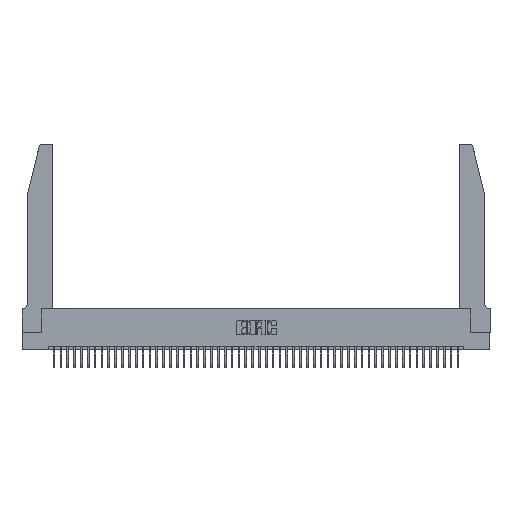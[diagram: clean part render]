
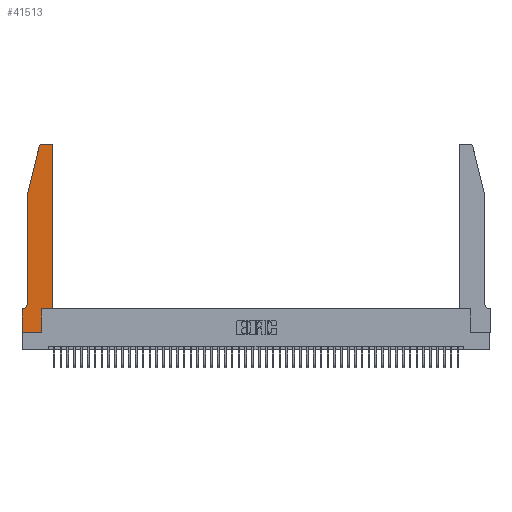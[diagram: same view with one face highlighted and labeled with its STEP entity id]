
A CAD part, top view. The second image highlights one B-rep face of the part: STEP entity #41513.
In plain terms, the highlighted planar face has unit normal (0, 0, 1).
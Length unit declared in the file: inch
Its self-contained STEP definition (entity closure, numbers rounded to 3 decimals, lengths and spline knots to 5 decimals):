
#330 = CIRCLE ( 'NONE', #25915, 0.07 ) ;
#775 = VECTOR ( 'NONE', #23107, 39.37008 ) ;
#2225 = VECTOR ( 'NONE', #41703, 39.37008 ) ;
#2553 = VERTEX_POINT ( 'NONE', #5997 ) ;
#3724 = CARTESIAN_POINT ( 'NONE',  ( 0., 0., 0.37 ) ) ;
#4008 = ORIENTED_EDGE ( 'NONE', *, *, #17469, .T. ) ;
#4079 = ORIENTED_EDGE ( 'NONE', *, *, #15821, .T. ) ;
#4320 = DIRECTION ( 'NONE',  ( 0., 0., 1. ) ) ;
#4356 = VERTEX_POINT ( 'NONE', #34598 ) ;
#4429 = PLANE ( 'NONE',  #10788 ) ;
#4528 = DIRECTION ( 'NONE',  ( -1., 0., 0. ) ) ;
#4863 = CARTESIAN_POINT ( 'NONE',  ( 0.0755, 2., 0.37 ) ) ;
#4899 = LINE ( 'NONE', #30300, #35871 ) ;
#5863 = DIRECTION ( 'NONE',  ( 0., 0., -1. ) ) ;
#5871 = EDGE_CURVE ( 'NONE', #2553, #21811, #7410, .T. ) ;
#5997 = CARTESIAN_POINT ( 'NONE',  ( 0.4205, 2.75, 0.37 ) ) ;
#6788 = VERTEX_POINT ( 'NONE', #37361 ) ;
#7410 = LINE ( 'NONE', #32541, #9270 ) ;
#7857 = EDGE_CURVE ( 'NONE', #38360, #44325, #42162, .T. ) ;
#8050 = LINE ( 'NONE', #15309, #49003 ) ;
#8825 = DIRECTION ( 'NONE',  ( -1., 0., 0. ) ) ;
#9270 = VECTOR ( 'NONE', #4528, 39.37008 ) ;
#9392 = ORIENTED_EDGE ( 'NONE', *, *, #22979, .T. ) ;
#10157 = CARTESIAN_POINT ( 'NONE',  ( 0.4505, 0.35, 0.37 ) ) ;
#10320 = EDGE_CURVE ( 'NONE', #40741, #44438, #4899, .T. ) ;
#10397 = VECTOR ( 'NONE', #37818, 39.37008 ) ;
#10788 = AXIS2_PLACEMENT_3D ( 'NONE', #47570, #27808, #16362 ) ;
#11617 = ORIENTED_EDGE ( 'NONE', *, *, #30626, .T. ) ;
#12096 = LINE ( 'NONE', #30519, #2225 ) ;
#12573 = ORIENTED_EDGE ( 'NONE', *, *, #26040, .T. ) ;
#13801 = DIRECTION ( 'NONE',  ( -0.239, -0.971, 0. ) ) ;
#14294 = AXIS2_PLACEMENT_3D ( 'NONE', #43527, #4320, #20237 ) ;
#15309 = CARTESIAN_POINT ( 'NONE',  ( 0.4505, 0.35, 0.37 ) ) ;
#15821 = EDGE_CURVE ( 'NONE', #4356, #38360, #24562, .T. ) ;
#16362 = DIRECTION ( 'NONE',  ( 1., 0., 0. ) ) ;
#16591 = EDGE_CURVE ( 'NONE', #6788, #2553, #18347, .T. ) ;
#16665 = CARTESIAN_POINT ( 'NONE',  ( 0., 0., 0.37 ) ) ;
#17469 = EDGE_CURVE ( 'NONE', #21811, #20927, #39288, .T. ) ;
#18170 = ORIENTED_EDGE ( 'NONE', *, *, #7857, .T. ) ;
#18347 = CIRCLE ( 'NONE', #14294, 0.03 ) ;
#19002 = CARTESIAN_POINT ( 'NONE',  ( 0.2865, 0., 0.37 ) ) ;
#19344 = LINE ( 'NONE', #49298, #39731 ) ;
#20237 = DIRECTION ( 'NONE',  ( 1., 0., 0. ) ) ;
#20921 = LINE ( 'NONE', #10157, #10397 ) ;
#20927 = VERTEX_POINT ( 'NONE', #37282 ) ;
#20932 = ORIENTED_EDGE ( 'NONE', *, *, #10320, .T. ) ;
#20933 = CARTESIAN_POINT ( 'NONE',  ( 0.0755, 0.35, 0.37 ) ) ;
#21811 = VERTEX_POINT ( 'NONE', #34122 ) ;
#22241 = DIRECTION ( 'NONE',  ( 1., 0., 0. ) ) ;
#22834 = DIRECTION ( 'NONE',  ( 0., 1., 0. ) ) ;
#22979 = EDGE_CURVE ( 'NONE', #24033, #25685, #30162, .T. ) ;
#23101 = DIRECTION ( 'NONE',  ( 1., 0., 0. ) ) ;
#23107 = DIRECTION ( 'NONE',  ( 0., -1., 0. ) ) ;
#24033 = VERTEX_POINT ( 'NONE', #4863 ) ;
#24562 = LINE ( 'NONE', #20933, #41231 ) ;
#25685 = VERTEX_POINT ( 'NONE', #32483 ) ;
#25721 = DIRECTION ( 'NONE',  ( 0., 0., 1. ) ) ;
#25801 = EDGE_CURVE ( 'NONE', #20927, #24033, #19344, .T. ) ;
#25915 = AXIS2_PLACEMENT_3D ( 'NONE', #37495, #5863, #45572 ) ;
#26040 = EDGE_CURVE ( 'NONE', #44438, #50279, #8050, .T. ) ;
#26434 = DIRECTION ( 'NONE',  ( 0., -1., 0. ) ) ;
#27808 = DIRECTION ( 'NONE',  ( 0., 0., 1. ) ) ;
#29791 = ORIENTED_EDGE ( 'NONE', *, *, #49824, .T. ) ;
#30077 = CARTESIAN_POINT ( 'NONE',  ( 0.0755, 2., 0.37 ) ) ;
#30162 = LINE ( 'NONE', #30077, #45552 ) ;
#30300 = CARTESIAN_POINT ( 'NONE',  ( 0.2865, 0.35, 0.37 ) ) ;
#30519 = CARTESIAN_POINT ( 'NONE',  ( 0., 0., 0.37 ) ) ;
#30626 = EDGE_CURVE ( 'NONE', #25685, #4356, #330, .T. ) ;
#32483 = CARTESIAN_POINT ( 'NONE',  ( 0.0755, 0.42, 0.37 ) ) ;
#32541 = CARTESIAN_POINT ( 'NONE',  ( 0.2605, 2.75, 0.37 ) ) ;
#34122 = CARTESIAN_POINT ( 'NONE',  ( 0.284, 2.75, 0.37 ) ) ;
#34598 = CARTESIAN_POINT ( 'NONE',  ( 0.0055, 0.35, 0.37 ) ) ;
#34716 = EDGE_CURVE ( 'NONE', #44325, #40741, #12096, .T. ) ;
#35328 = ORIENTED_EDGE ( 'NONE', *, *, #34716, .T. ) ;
#35871 = VECTOR ( 'NONE', #22834, 39.37008 ) ;
#37118 = CARTESIAN_POINT ( 'NONE',  ( 0., 0.35, 0.37 ) ) ;
#37282 = CARTESIAN_POINT ( 'NONE',  ( 0.25487, 2.72718, 0.37 ) ) ;
#37361 = CARTESIAN_POINT ( 'NONE',  ( 0.4505, 2.72, 0.37 ) ) ;
#37495 = CARTESIAN_POINT ( 'NONE',  ( 0.0055, 0.42, 0.37 ) ) ;
#37624 = CARTESIAN_POINT ( 'NONE',  ( 0.284, 2.72, 0.37 ) ) ;
#37818 = DIRECTION ( 'NONE',  ( 0., 1., 0. ) ) ;
#38360 = VERTEX_POINT ( 'NONE', #37118 ) ;
#38824 = ORIENTED_EDGE ( 'NONE', *, *, #25801, .T. ) ;
#39288 = CIRCLE ( 'NONE', #41593, 0.03 ) ;
#39731 = VECTOR ( 'NONE', #13801, 39.37008 ) ;
#40490 = CARTESIAN_POINT ( 'NONE',  ( 0.2865, 0.35, 0.37 ) ) ;
#40741 = VERTEX_POINT ( 'NONE', #19002 ) ;
#41231 = VECTOR ( 'NONE', #8825, 39.37008 ) ;
#41513 = ADVANCED_FACE ( 'NONE', ( #47715 ), #4429, .T. ) ;
#41593 = AXIS2_PLACEMENT_3D ( 'NONE', #37624, #25721, #22241 ) ;
#41703 = DIRECTION ( 'NONE',  ( 1., 0., 0. ) ) ;
#42162 = LINE ( 'NONE', #3724, #775 ) ;
#42391 = ORIENTED_EDGE ( 'NONE', *, *, #16591, .T. ) ;
#42425 = ORIENTED_EDGE ( 'NONE', *, *, #5871, .T. ) ;
#43527 = CARTESIAN_POINT ( 'NONE',  ( 0.4205, 2.72, 0.37 ) ) ;
#44300 = CARTESIAN_POINT ( 'NONE',  ( 0.4505, 0.35, 0.37 ) ) ;
#44325 = VERTEX_POINT ( 'NONE', #16665 ) ;
#44438 = VERTEX_POINT ( 'NONE', #40490 ) ;
#45552 = VECTOR ( 'NONE', #26434, 39.37008 ) ;
#45572 = DIRECTION ( 'NONE',  ( -1., 0., 0. ) ) ;
#47290 = EDGE_LOOP ( 'NONE', ( #42425, #4008, #38824, #9392, #11617, #4079, #18170, #35328, #20932, #12573, #29791, #42391 ) ) ;
#47570 = CARTESIAN_POINT ( 'NONE',  ( 0., 0.35, 0.37 ) ) ;
#47715 = FACE_OUTER_BOUND ( 'NONE', #47290, .T. ) ;
#49003 = VECTOR ( 'NONE', #23101, 39.37008 ) ;
#49298 = CARTESIAN_POINT ( 'NONE',  ( 0.0755, 2., 0.37 ) ) ;
#49824 = EDGE_CURVE ( 'NONE', #50279, #6788, #20921, .T. ) ;
#50279 = VERTEX_POINT ( 'NONE', #44300 ) ;
